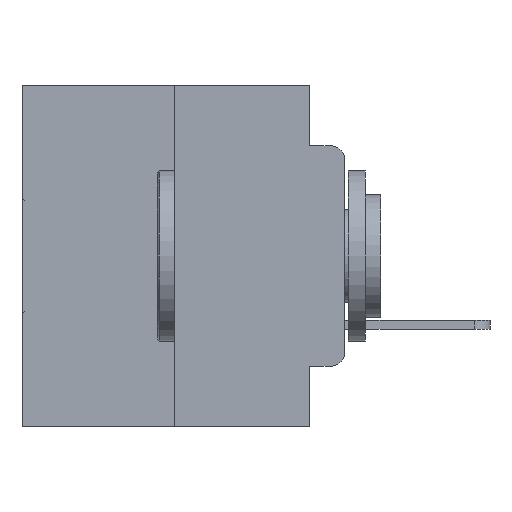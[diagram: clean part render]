
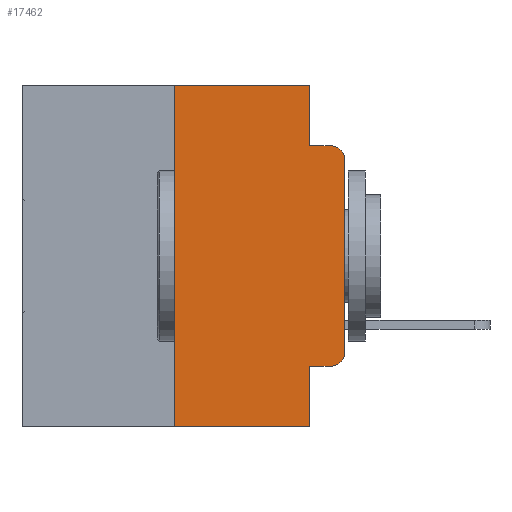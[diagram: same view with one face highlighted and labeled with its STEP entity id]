
A CAD part, left-side view. The second image highlights one B-rep face of the part: STEP entity #17462.
In plain terms, the highlighted planar face has unit normal (-1, 0, 0).
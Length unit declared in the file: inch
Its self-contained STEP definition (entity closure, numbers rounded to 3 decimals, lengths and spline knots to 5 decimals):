
#162 = VERTEX_POINT ( 'NONE', #2314 ) ;
#446 = VERTEX_POINT ( 'NONE', #25849 ) ;
#786 = ORIENTED_EDGE ( 'NONE', *, *, #29457, .F. ) ;
#1104 = ORIENTED_EDGE ( 'NONE', *, *, #24772, .T. ) ;
#2025 = CARTESIAN_POINT ( 'NONE',  ( 0., 0.051, 0. ) ) ;
#2314 = CARTESIAN_POINT ( 'NONE',  ( 0., 0., -0.1085 ) ) ;
#2440 = EDGE_CURVE ( 'NONE', #26306, #26699, #24716, .T. ) ;
#2753 = VERTEX_POINT ( 'NONE', #12636 ) ;
#4168 = VECTOR ( 'NONE', #5044, 39.37008 ) ;
#5044 = DIRECTION ( 'NONE',  ( 0., -1., 0. ) ) ;
#5082 = DIRECTION ( 'NONE',  ( 0., 0., -1. ) ) ;
#5249 = VECTOR ( 'NONE', #8079, 39.37008 ) ;
#5901 = DIRECTION ( 'NONE',  ( 0., 0., -1. ) ) ;
#6357 = AXIS2_PLACEMENT_3D ( 'NONE', #18711, #18318, #18414 ) ;
#6421 = ORIENTED_EDGE ( 'NONE', *, *, #23232, .F. ) ;
#6551 = LINE ( 'NONE', #2025, #24483 ) ;
#7018 = CIRCLE ( 'NONE', #7832, 0.02 ) ;
#7308 = VERTEX_POINT ( 'NONE', #14403 ) ;
#7832 = AXIS2_PLACEMENT_3D ( 'NONE', #24457, #10496, #5901 ) ;
#7989 = CARTESIAN_POINT ( 'NONE',  ( 0., 0.25, 0. ) ) ;
#8079 = DIRECTION ( 'NONE',  ( 0., -1., 0. ) ) ;
#8170 = VERTEX_POINT ( 'NONE', #22563 ) ;
#8400 = PLANE ( 'NONE',  #28521 ) ;
#8713 = DIRECTION ( 'NONE',  ( 1., 0., 0. ) ) ;
#9180 = DIRECTION ( 'NONE',  ( 0., 0., 1. ) ) ;
#9951 = VECTOR ( 'NONE', #9180, 39.37008 ) ;
#10496 = DIRECTION ( 'NONE',  ( -1., 0., 0. ) ) ;
#10988 = FACE_OUTER_BOUND ( 'NONE', #13426, .T. ) ;
#12208 = DIRECTION ( 'NONE',  ( 0., -1., 0. ) ) ;
#12581 = LINE ( 'NONE', #24701, #5249 ) ;
#12636 = CARTESIAN_POINT ( 'NONE',  ( 0., 0., -0.3915 ) ) ;
#13426 = EDGE_LOOP ( 'NONE', ( #15028, #1104, #6421, #786, #14967, #25917, #23772, #25521, #18771, #28482 ) ) ;
#13816 = VECTOR ( 'NONE', #12208, 39.37008 ) ;
#13822 = DIRECTION ( 'NONE',  ( 0., 0., -1. ) ) ;
#14403 = CARTESIAN_POINT ( 'NONE',  ( 0., 0.051, 0. ) ) ;
#14744 = EDGE_CURVE ( 'NONE', #19537, #22820, #15204, .T. ) ;
#14778 = CARTESIAN_POINT ( 'NONE',  ( 0., 0.473, 0. ) ) ;
#14967 = ORIENTED_EDGE ( 'NONE', *, *, #18577, .F. ) ;
#15028 = ORIENTED_EDGE ( 'NONE', *, *, #24356, .T. ) ;
#15204 = LINE ( 'NONE', #27385, #26965 ) ;
#15610 = EDGE_CURVE ( 'NONE', #22820, #2753, #24778, .T. ) ;
#16120 = VECTOR ( 'NONE', #5082, 39.37008 ) ;
#16138 = CARTESIAN_POINT ( 'NONE',  ( 0., 0., 0. ) ) ;
#16251 = CARTESIAN_POINT ( 'NONE',  ( 0., 0.25, 0. ) ) ;
#16568 = DIRECTION ( 'NONE',  ( 0., 0., -1. ) ) ;
#17462 = ADVANCED_FACE ( 'NONE', ( #10988 ), #8400, .F. ) ;
#17864 = DIRECTION ( 'NONE',  ( 0., -1., 0. ) ) ;
#18011 = CARTESIAN_POINT ( 'NONE',  ( 0., 0.051, 0. ) ) ;
#18318 = DIRECTION ( 'NONE',  ( -1., 0., 0. ) ) ;
#18414 = DIRECTION ( 'NONE',  ( 0., 0., -1. ) ) ;
#18577 = EDGE_CURVE ( 'NONE', #26699, #7308, #22656, .T. ) ;
#18711 = CARTESIAN_POINT ( 'NONE',  ( 0., 0.02, -0.3915 ) ) ;
#18771 = ORIENTED_EDGE ( 'NONE', *, *, #14744, .T. ) ;
#19210 = CARTESIAN_POINT ( 'NONE',  ( 0., 0.051, -0.0885 ) ) ;
#19537 = VERTEX_POINT ( 'NONE', #27869 ) ;
#20143 = EDGE_CURVE ( 'NONE', #26306, #446, #12581, .T. ) ;
#20546 = CARTESIAN_POINT ( 'NONE',  ( 0., 0.25, -0.5 ) ) ;
#21009 = DIRECTION ( 'NONE',  ( 0., 0., 1. ) ) ;
#21885 = VERTEX_POINT ( 'NONE', #22326 ) ;
#22078 = EDGE_CURVE ( 'NONE', #19537, #446, #29324, .T. ) ;
#22326 = CARTESIAN_POINT ( 'NONE',  ( 0., 0.051, -0.0885 ) ) ;
#22563 = CARTESIAN_POINT ( 'NONE',  ( 0., 0.02, -0.0885 ) ) ;
#22656 = LINE ( 'NONE', #14778, #13816 ) ;
#22772 = CARTESIAN_POINT ( 'NONE',  ( 0., 0.473, 0. ) ) ;
#22820 = VERTEX_POINT ( 'NONE', #27646 ) ;
#23232 = EDGE_CURVE ( 'NONE', #21885, #8170, #24698, .T. ) ;
#23565 = LINE ( 'NONE', #16138, #9951 ) ;
#23772 = ORIENTED_EDGE ( 'NONE', *, *, #20143, .T. ) ;
#24322 = VECTOR ( 'NONE', #21009, 39.37008 ) ;
#24356 = EDGE_CURVE ( 'NONE', #2753, #162, #23565, .T. ) ;
#24457 = CARTESIAN_POINT ( 'NONE',  ( 0., 0.02, -0.1085 ) ) ;
#24483 = VECTOR ( 'NONE', #13822, 39.37008 ) ;
#24698 = LINE ( 'NONE', #19210, #4168 ) ;
#24701 = CARTESIAN_POINT ( 'NONE',  ( 0., 0.473, -0.5 ) ) ;
#24716 = LINE ( 'NONE', #16251, #24322 ) ;
#24772 = EDGE_CURVE ( 'NONE', #162, #8170, #7018, .T. ) ;
#24778 = CIRCLE ( 'NONE', #6357, 0.02 ) ;
#25521 = ORIENTED_EDGE ( 'NONE', *, *, #22078, .F. ) ;
#25849 = CARTESIAN_POINT ( 'NONE',  ( 0., 0.051, -0.5 ) ) ;
#25917 = ORIENTED_EDGE ( 'NONE', *, *, #2440, .F. ) ;
#26306 = VERTEX_POINT ( 'NONE', #20546 ) ;
#26699 = VERTEX_POINT ( 'NONE', #7989 ) ;
#26965 = VECTOR ( 'NONE', #17864, 39.37008 ) ;
#27385 = CARTESIAN_POINT ( 'NONE',  ( 0., 0.051, -0.4115 ) ) ;
#27646 = CARTESIAN_POINT ( 'NONE',  ( 0., 0.02, -0.4115 ) ) ;
#27869 = CARTESIAN_POINT ( 'NONE',  ( 0., 0.051, -0.4115 ) ) ;
#28482 = ORIENTED_EDGE ( 'NONE', *, *, #15610, .T. ) ;
#28521 = AXIS2_PLACEMENT_3D ( 'NONE', #22772, #8713, #16568 ) ;
#29324 = LINE ( 'NONE', #18011, #16120 ) ;
#29457 = EDGE_CURVE ( 'NONE', #7308, #21885, #6551, .T. ) ;
